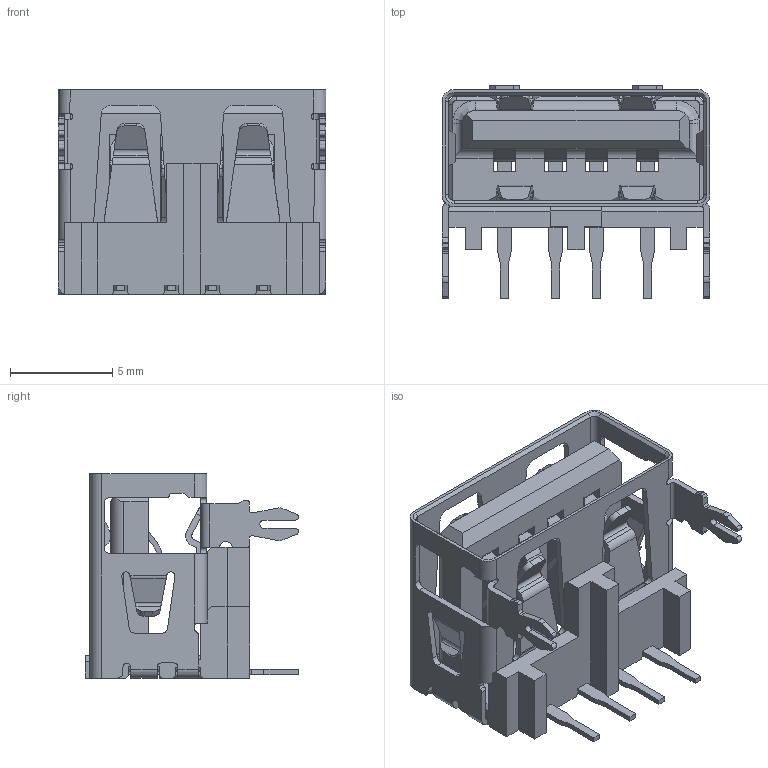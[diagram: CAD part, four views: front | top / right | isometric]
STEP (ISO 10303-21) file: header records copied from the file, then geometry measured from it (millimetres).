
FILE_DESCRIPTION (( 'STEP AP214' ), '1' );
FILE_NAME ('690A104-123-621.STEP', '2021-01-18T16:08:55', ( '' ), ( '' ), 'SwSTEP 2.0', 'SolidWorks 2020', '' );
FILE_SCHEMA (( 'AUTOMOTIVE_DESIGN' ));
Length unit declared in the file: millimetre
Products named in the file (4): Shell 690A104-123-621; Contact 690A104-123-621; Insulator 690A104-123-621; 690A104-123-621
Assembly tree (6 placements, depth 2):
  690A104-123-621
    Insulator 690A104-123-621
    Contact 690A104-123-621  x4
    Shell 690A104-123-621
Bounding box: 13.1 x 10.43 x 10 mm (x, y, z)
Volume: 326.8 mm3; surface area: 1425.3 mm2
Topology: 6 solids, 6 shells, 949 faces, 2770 edges, 1820 vertices
Faces by surface type: plane 599, cylinder 232, bspline 112, cone 6
Entity records: 24133 total; most frequent: CARTESIAN_POINT 6067, ORIENTED_EDGE 4046, DIRECTION 3357, EDGE_CURVE 2023, VECTOR 1517, LINE 1517, VERTEX_POINT 1328, AXIS2_PLACEMENT_3D 920
